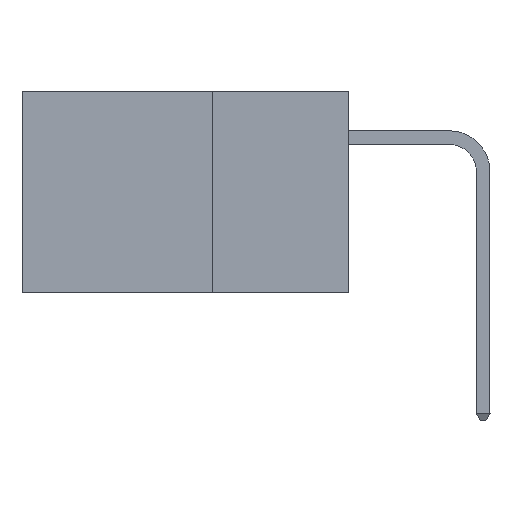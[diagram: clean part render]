
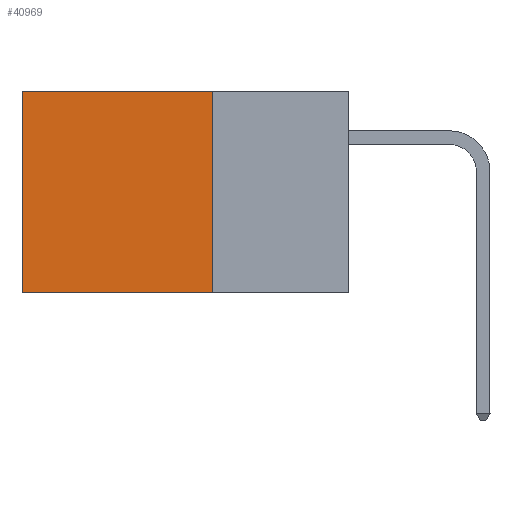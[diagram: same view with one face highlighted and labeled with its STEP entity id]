
A CAD part, left-side view. The second image highlights one B-rep face of the part: STEP entity #40969.
In plain terms, the highlighted planar face has unit normal (-1, 0, 0).
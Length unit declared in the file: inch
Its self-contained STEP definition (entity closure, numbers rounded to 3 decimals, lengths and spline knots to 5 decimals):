
#1276 = VERTEX_POINT ( 'NONE', #39054 ) ;
#2249 = LINE ( 'NONE', #9043, #40436 ) ;
#3615 = LINE ( 'NONE', #37758, #38538 ) ;
#7745 = EDGE_CURVE ( 'NONE', #11974, #28279, #20166, .T. ) ;
#9043 = CARTESIAN_POINT ( 'NONE',  ( 0.2875, 0.25, 0. ) ) ;
#10576 = CARTESIAN_POINT ( 'NONE',  ( 0.2875, 0.25, 0. ) ) ;
#11145 = ORIENTED_EDGE ( 'NONE', *, *, #7745, .T. ) ;
#11974 = VERTEX_POINT ( 'NONE', #42213 ) ;
#12898 = VECTOR ( 'NONE', #19941, 39.37008 ) ;
#12949 = CARTESIAN_POINT ( 'NONE',  ( 0.2875, 0.6, 0. ) ) ;
#13416 = DIRECTION ( 'NONE',  ( 1., 0., 0. ) ) ;
#13613 = EDGE_CURVE ( 'NONE', #1276, #38417, #42908, .T. ) ;
#13778 = CARTESIAN_POINT ( 'NONE',  ( 0.2875, 0.25, -0.37 ) ) ;
#15556 = EDGE_LOOP ( 'NONE', ( #11145, #29809, #25739, #37209 ) ) ;
#16609 = VECTOR ( 'NONE', #19081, 39.37008 ) ;
#18029 = DIRECTION ( 'NONE',  ( 0., 1., 0. ) ) ;
#19081 = DIRECTION ( 'NONE',  ( 0., 0., -1. ) ) ;
#19941 = DIRECTION ( 'NONE',  ( 0., 0., -1. ) ) ;
#19978 = DIRECTION ( 'NONE',  ( 0., 0., -1. ) ) ;
#20166 = LINE ( 'NONE', #12949, #12898 ) ;
#23263 = PLANE ( 'NONE',  #41276 ) ;
#23921 = FACE_OUTER_BOUND ( 'NONE', #15556, .T. ) ;
#25739 = ORIENTED_EDGE ( 'NONE', *, *, #13613, .F. ) ;
#25874 = CARTESIAN_POINT ( 'NONE',  ( 0.2875, 0.25, 0. ) ) ;
#28279 = VERTEX_POINT ( 'NONE', #35311 ) ;
#29809 = ORIENTED_EDGE ( 'NONE', *, *, #41835, .F. ) ;
#30525 = DIRECTION ( 'NONE',  ( 0., 1., 0. ) ) ;
#34192 = EDGE_CURVE ( 'NONE', #1276, #11974, #2249, .T. ) ;
#35311 = CARTESIAN_POINT ( 'NONE',  ( 0.2875, 0.6, -0.37 ) ) ;
#37209 = ORIENTED_EDGE ( 'NONE', *, *, #34192, .T. ) ;
#37758 = CARTESIAN_POINT ( 'NONE',  ( 0.2875, 0.25, -0.37 ) ) ;
#38417 = VERTEX_POINT ( 'NONE', #13778 ) ;
#38538 = VECTOR ( 'NONE', #30525, 39.37008 ) ;
#39054 = CARTESIAN_POINT ( 'NONE',  ( 0.2875, 0.25, 0. ) ) ;
#40436 = VECTOR ( 'NONE', #18029, 39.37008 ) ;
#40969 = ADVANCED_FACE ( 'NONE', ( #23921 ), #23263, .F. ) ;
#41276 = AXIS2_PLACEMENT_3D ( 'NONE', #10576, #13416, #19978 ) ;
#41835 = EDGE_CURVE ( 'NONE', #38417, #28279, #3615, .T. ) ;
#42213 = CARTESIAN_POINT ( 'NONE',  ( 0.2875, 0.6, 0. ) ) ;
#42908 = LINE ( 'NONE', #25874, #16609 ) ;
